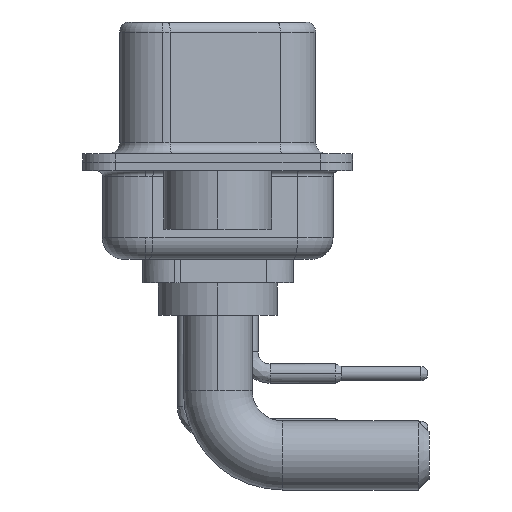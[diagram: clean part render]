
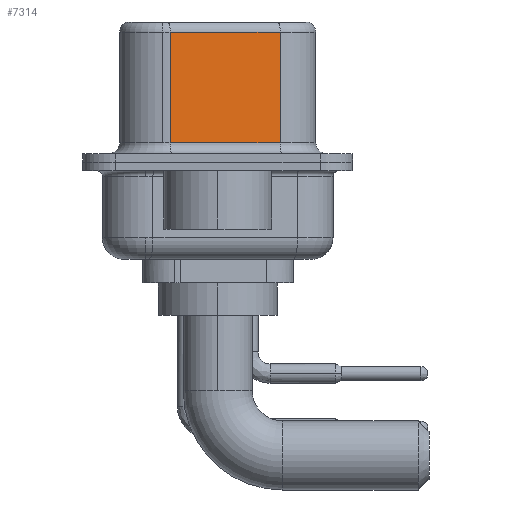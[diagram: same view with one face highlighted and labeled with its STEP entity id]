
A CAD part, left-side view. The second image highlights one B-rep face of the part: STEP entity #7314.
In plain terms, the highlighted planar face has unit normal (-0.985, -0.174, 0).
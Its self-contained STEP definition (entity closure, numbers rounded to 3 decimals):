
#336 = FACE_OUTER_BOUND ( 'NONE', #12483, .T. ) ;
#415 = LINE ( 'NONE', #12602, #16226 ) ;
#542 = CARTESIAN_POINT ( 'NONE',  ( 3.68, 2.203, 0.9 ) ) ;
#1777 = CARTESIAN_POINT ( 'NONE',  ( 3.68, 2.203, 6.02 ) ) ;
#2853 = ORIENTED_EDGE ( 'NONE', *, *, #20463, .T. ) ;
#4061 = LINE ( 'NONE', #7917, #14118 ) ;
#5879 = LINE ( 'NONE', #21442, #15905 ) ;
#6323 = CARTESIAN_POINT ( 'NONE',  ( 4.58, -2.897, 6.02 ) ) ;
#7314 = ADVANCED_FACE ( 'NONE', ( #336 ), #21143, .F. ) ;
#7369 = VERTEX_POINT ( 'NONE', #542 ) ;
#7917 = CARTESIAN_POINT ( 'NONE',  ( 4.58, -2.897, 6.52 ) ) ;
#9100 = DIRECTION ( 'NONE',  ( 0.985, 0.174, 0. ) ) ;
#9202 = DIRECTION ( 'NONE',  ( -0.174, 0.985, 0. ) ) ;
#10463 = VERTEX_POINT ( 'NONE', #1777 ) ;
#10521 = CARTESIAN_POINT ( 'NONE',  ( 4.58, -2.897, 0.9 ) ) ;
#10853 = CARTESIAN_POINT ( 'NONE',  ( 4.58, -2.897, 0.9 ) ) ;
#12483 = EDGE_LOOP ( 'NONE', ( #17951, #13569, #12720, #2853 ) ) ;
#12506 = CARTESIAN_POINT ( 'NONE',  ( 4.58, -2.897, 6.52 ) ) ;
#12602 = CARTESIAN_POINT ( 'NONE',  ( 4.58, -2.897, 6.02 ) ) ;
#12720 = ORIENTED_EDGE ( 'NONE', *, *, #20086, .T. ) ;
#13569 = ORIENTED_EDGE ( 'NONE', *, *, #15048, .T. ) ;
#14118 = VECTOR ( 'NONE', #21546, 1000. ) ;
#15048 = EDGE_CURVE ( 'NONE', #18113, #10463, #415, .T. ) ;
#15905 = VECTOR ( 'NONE', #18150, 1000. ) ;
#16226 = VECTOR ( 'NONE', #16238, 1000. ) ;
#16238 = DIRECTION ( 'NONE',  ( -0.174, 0.985, 0. ) ) ;
#17951 = ORIENTED_EDGE ( 'NONE', *, *, #20185, .F. ) ;
#18113 = VERTEX_POINT ( 'NONE', #6323 ) ;
#18150 = DIRECTION ( 'NONE',  ( 0., 0., -1. ) ) ;
#19177 = VECTOR ( 'NONE', #21088, 1000. ) ;
#19823 = AXIS2_PLACEMENT_3D ( 'NONE', #12506, #9100, #9202 ) ;
#20086 = EDGE_CURVE ( 'NONE', #10463, #7369, #5879, .T. ) ;
#20185 = EDGE_CURVE ( 'NONE', #18113, #20567, #4061, .T. ) ;
#20463 = EDGE_CURVE ( 'NONE', #7369, #20567, #21187, .T. ) ;
#20567 = VERTEX_POINT ( 'NONE', #10853 ) ;
#21088 = DIRECTION ( 'NONE',  ( 0.174, -0.985, 0. ) ) ;
#21143 = PLANE ( 'NONE',  #19823 ) ;
#21187 = LINE ( 'NONE', #10521, #19177 ) ;
#21442 = CARTESIAN_POINT ( 'NONE',  ( 3.68, 2.203, 6.52 ) ) ;
#21546 = DIRECTION ( 'NONE',  ( 0., 0., -1. ) ) ;
